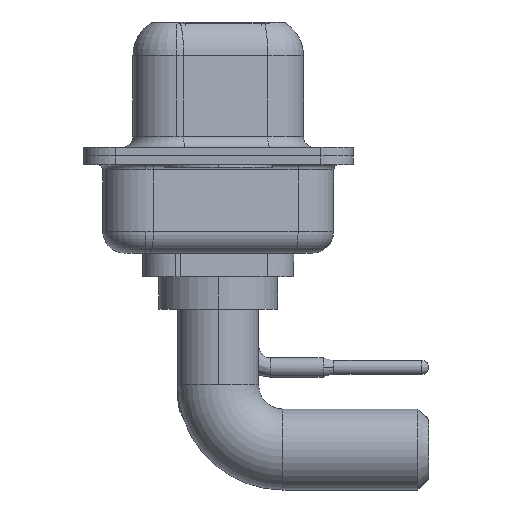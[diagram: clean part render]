
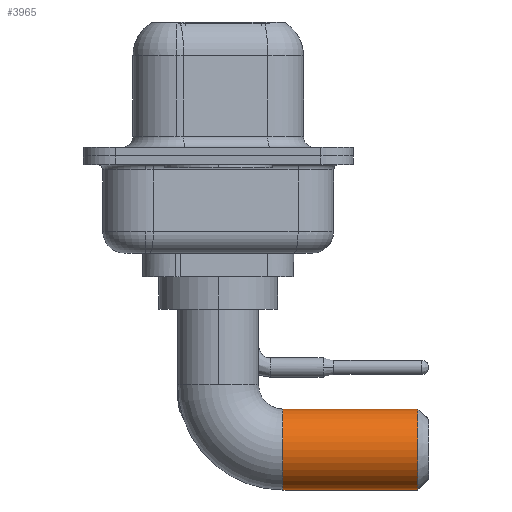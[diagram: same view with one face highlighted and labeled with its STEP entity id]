
A CAD part, left-side view. The second image highlights one B-rep face of the part: STEP entity #3965.
In plain terms, the highlighted cylindrical face has radius 1.875 mm (diameter 3.75 mm), a partial arc.
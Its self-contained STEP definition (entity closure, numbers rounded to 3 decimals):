
#401 = DIRECTION ( 'NONE',  ( 0., -1., 0. ) ) ;
#603 = CIRCLE ( 'NONE', #10374, 1.875 ) ;
#732 = AXIS2_PLACEMENT_3D ( 'NONE', #9255, #919, #9179 ) ;
#919 = DIRECTION ( 'NONE',  ( 0., -1., 0. ) ) ;
#1216 = VECTOR ( 'NONE', #401, 1000. ) ;
#1824 = CARTESIAN_POINT ( 'NONE',  ( 0., -3., -4.625 ) ) ;
#2404 = CARTESIAN_POINT ( 'NONE',  ( 0., -3., -4.625 ) ) ;
#3223 = VERTEX_POINT ( 'NONE', #7372 ) ;
#3437 = ORIENTED_EDGE ( 'NONE', *, *, #9829, .T. ) ;
#3854 = CARTESIAN_POINT ( 'NONE',  ( 0., -3., -6.5 ) ) ;
#3965 = ADVANCED_FACE ( 'NONE', ( #10555 ), #8093, .T. ) ;
#4620 = EDGE_CURVE ( 'NONE', #3223, #6775, #603, .T. ) ;
#4792 = VERTEX_POINT ( 'NONE', #2404 ) ;
#4930 = DIRECTION ( 'NONE',  ( -1., 0., 0. ) ) ;
#5258 = ORIENTED_EDGE ( 'NONE', *, *, #9691, .F. ) ;
#5388 = VERTEX_POINT ( 'NONE', #14190 ) ;
#5634 = ORIENTED_EDGE ( 'NONE', *, *, #10491, .T. ) ;
#6775 = VERTEX_POINT ( 'NONE', #7345 ) ;
#7013 = DIRECTION ( 'NONE',  ( 0., 1., 0. ) ) ;
#7345 = CARTESIAN_POINT ( 'NONE',  ( 0., -9.25, -4.625 ) ) ;
#7372 = CARTESIAN_POINT ( 'NONE',  ( 0., -9.25, -8.375 ) ) ;
#7575 = LINE ( 'NONE', #10890, #1216 ) ;
#7758 = VECTOR ( 'NONE', #10516, 1000. ) ;
#8093 = CYLINDRICAL_SURFACE ( 'NONE', #732, 1.875 ) ;
#8748 = AXIS2_PLACEMENT_3D ( 'NONE', #3854, #10595, #4930 ) ;
#8868 = EDGE_LOOP ( 'NONE', ( #5258, #3437, #5634, #14998 ) ) ;
#9179 = DIRECTION ( 'NONE',  ( 0., 0., -1. ) ) ;
#9255 = CARTESIAN_POINT ( 'NONE',  ( 0., -3., -6.5 ) ) ;
#9391 = DIRECTION ( 'NONE',  ( 0., 0., -1. ) ) ;
#9463 = CARTESIAN_POINT ( 'NONE',  ( 0., -9.25, -6.5 ) ) ;
#9691 = EDGE_CURVE ( 'NONE', #4792, #6775, #14799, .T. ) ;
#9829 = EDGE_CURVE ( 'NONE', #4792, #5388, #13627, .T. ) ;
#10374 = AXIS2_PLACEMENT_3D ( 'NONE', #9463, #7013, #9391 ) ;
#10491 = EDGE_CURVE ( 'NONE', #5388, #3223, #7575, .T. ) ;
#10516 = DIRECTION ( 'NONE',  ( 0., -1., 0. ) ) ;
#10555 = FACE_OUTER_BOUND ( 'NONE', #8868, .T. ) ;
#10595 = DIRECTION ( 'NONE',  ( 0., -1., 0. ) ) ;
#10890 = CARTESIAN_POINT ( 'NONE',  ( 0., -3., -8.375 ) ) ;
#13627 = CIRCLE ( 'NONE', #8748, 1.875 ) ;
#14190 = CARTESIAN_POINT ( 'NONE',  ( 0., -3., -8.375 ) ) ;
#14799 = LINE ( 'NONE', #1824, #7758 ) ;
#14998 = ORIENTED_EDGE ( 'NONE', *, *, #4620, .T. ) ;
